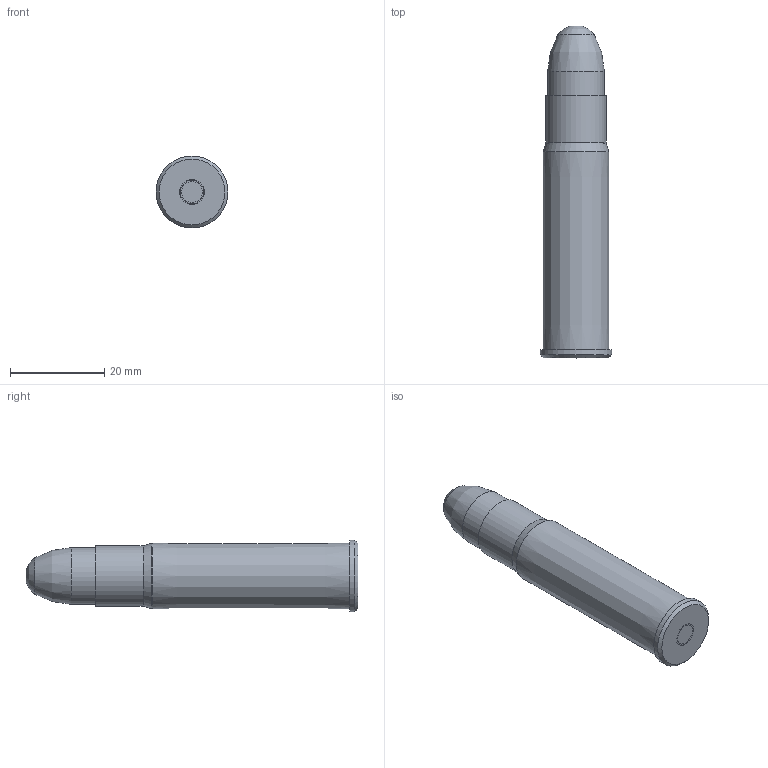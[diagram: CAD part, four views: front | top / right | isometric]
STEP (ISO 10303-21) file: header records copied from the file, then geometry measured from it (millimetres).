
FILE_DESCRIPTION((''),'2;1');
FILE_NAME('475 TURNBULL.stp','2012-11-30T12:29:45',('AGARRETT'),(''),'Autodesk Inventor 2012','Autodesk Inventor 2012','');
FILE_SCHEMA(('AUTOMOTIVE_DESIGN { 1 0 10303 214 1 1 1 1 }'));
Length unit declared in the file: inch
Products named in the file (4): iLogic Cartridge; Rimmed Bottleneck; iLogic RN Bullet; PRIMER
Assembly tree (3 placements, depth 2):
  iLogic Cartridge
    Rimmed Bottleneck
    iLogic RN Bullet
    PRIMER
Bounding box: 15.29 x 70.61 x 15.29 mm (x, y, z)
Volume: 10954.3 mm3; surface area: 4001.2 mm2
Topology: 3 solids, 3 shells, 27 faces, 41 edges, 24 vertices
Faces by surface type: plane 10, cylinder 7, torus 5, cone 3, bspline 2
Full cylindrical faces by diameter (mm): 1.778 x1, 4.445 x1, 5.08 x1, 5.334 x1, 12.065 x1, 12.776 x1, 15.291 x1
Entity records: 704 total; most frequent: CARTESIAN_POINT 134, DIRECTION 112, AXIS2_PLACEMENT_3D 56, ORIENTED_EDGE 48, EDGE_LOOP 48, FACE_OUTER_BOUND 27, ADVANCED_FACE 27, VERTEX_POINT 24
